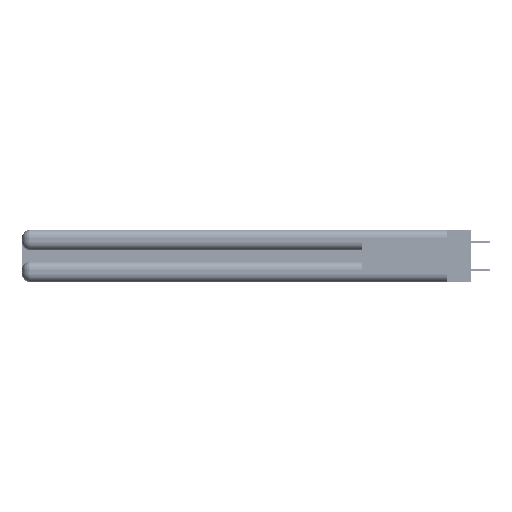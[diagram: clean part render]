
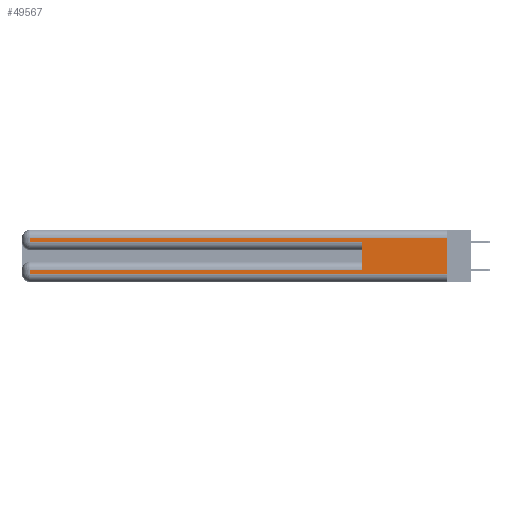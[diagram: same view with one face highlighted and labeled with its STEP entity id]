
A CAD part, left-side view. The second image highlights one B-rep face of the part: STEP entity #49567.
In plain terms, the highlighted planar face has unit normal (-1, 0, 0).
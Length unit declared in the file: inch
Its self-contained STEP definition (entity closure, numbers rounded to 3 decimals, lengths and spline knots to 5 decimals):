
#527 = VERTEX_POINT ( 'NONE', #23845 ) ;
#1686 = DIRECTION ( 'NONE',  ( 0., 1., 0. ) ) ;
#2031 = FACE_OUTER_BOUND ( 'NONE', #20656, .T. ) ;
#5132 = DIRECTION ( 'NONE',  ( 0., -1., 0. ) ) ;
#6232 = LINE ( 'NONE', #6499, #11793 ) ;
#6499 = CARTESIAN_POINT ( 'NONE',  ( 0., 0., 0.31 ) ) ;
#7122 = VERTEX_POINT ( 'NONE', #25408 ) ;
#7127 = CARTESIAN_POINT ( 'NONE',  ( 0., 0., 0.37 ) ) ;
#7706 = DIRECTION ( 'NONE',  ( 0., 1., 0. ) ) ;
#8809 = LINE ( 'NONE', #55264, #35926 ) ;
#9026 = ORIENTED_EDGE ( 'NONE', *, *, #32022, .F. ) ;
#10526 = CARTESIAN_POINT ( 'NONE',  ( 0., 0.6, 0.285 ) ) ;
#11391 = ORIENTED_EDGE ( 'NONE', *, *, #53715, .T. ) ;
#11528 = LINE ( 'NONE', #23981, #28652 ) ;
#11734 = VECTOR ( 'NONE', #44855, 39.37008 ) ;
#11793 = VECTOR ( 'NONE', #1686, 39.37008 ) ;
#11884 = CARTESIAN_POINT ( 'NONE',  ( 0., 0., 0.37 ) ) ;
#12085 = VERTEX_POINT ( 'NONE', #18252 ) ;
#12910 = LINE ( 'NONE', #13932, #48203 ) ;
#13932 = CARTESIAN_POINT ( 'NONE',  ( 0., 0., 0.285 ) ) ;
#14087 = CARTESIAN_POINT ( 'NONE',  ( 0., 2.94, 0.085 ) ) ;
#14174 = CARTESIAN_POINT ( 'NONE',  ( 0., 0., 0.06 ) ) ;
#14589 = CARTESIAN_POINT ( 'NONE',  ( 0., 0.6, 0.145 ) ) ;
#15603 = LINE ( 'NONE', #55485, #38259 ) ;
#17709 = EDGE_CURVE ( 'NONE', #24089, #52667, #27595, .T. ) ;
#18252 = CARTESIAN_POINT ( 'NONE',  ( 0., 2.94, 0.06 ) ) ;
#20656 = EDGE_LOOP ( 'NONE', ( #9026, #34301, #11391, #23757, #26245, #27391, #32848, #41834 ) ) ;
#21561 = VERTEX_POINT ( 'NONE', #14087 ) ;
#22673 = CARTESIAN_POINT ( 'NONE',  ( 0., 0.6, 0.085 ) ) ;
#23757 = ORIENTED_EDGE ( 'NONE', *, *, #49442, .T. ) ;
#23845 = CARTESIAN_POINT ( 'NONE',  ( 0., 2.94, 0.285 ) ) ;
#23981 = CARTESIAN_POINT ( 'NONE',  ( 0., 2.94, 0.37 ) ) ;
#24077 = EDGE_CURVE ( 'NONE', #12085, #7122, #26361, .T. ) ;
#24089 = VERTEX_POINT ( 'NONE', #22673 ) ;
#25141 = CARTESIAN_POINT ( 'NONE',  ( 0., 0., 0.31 ) ) ;
#25408 = CARTESIAN_POINT ( 'NONE',  ( 0., 0., 0.06 ) ) ;
#26245 = ORIENTED_EDGE ( 'NONE', *, *, #17709, .F. ) ;
#26361 = LINE ( 'NONE', #14174, #27383 ) ;
#27383 = VECTOR ( 'NONE', #5132, 39.37008 ) ;
#27391 = ORIENTED_EDGE ( 'NONE', *, *, #33366, .T. ) ;
#27595 = LINE ( 'NONE', #14589, #11734 ) ;
#28627 = PLANE ( 'NONE',  #33779 ) ;
#28652 = VECTOR ( 'NONE', #50009, 39.37008 ) ;
#29133 = DIRECTION ( 'NONE',  ( 0., 0., -1. ) ) ;
#31171 = DIRECTION ( 'NONE',  ( 0., -1., 0. ) ) ;
#32022 = EDGE_CURVE ( 'NONE', #35459, #7122, #50654, .T. ) ;
#32848 = ORIENTED_EDGE ( 'NONE', *, *, #47241, .T. ) ;
#33366 = EDGE_CURVE ( 'NONE', #24089, #21561, #8809, .T. ) ;
#33779 = AXIS2_PLACEMENT_3D ( 'NONE', #7127, #53837, #41633 ) ;
#34301 = ORIENTED_EDGE ( 'NONE', *, *, #37969, .T. ) ;
#35459 = VERTEX_POINT ( 'NONE', #25141 ) ;
#35926 = VECTOR ( 'NONE', #7706, 39.37008 ) ;
#37969 = EDGE_CURVE ( 'NONE', #35459, #51095, #6232, .T. ) ;
#38259 = VECTOR ( 'NONE', #51238, 39.37008 ) ;
#41633 = DIRECTION ( 'NONE',  ( 0., 0., -1. ) ) ;
#41834 = ORIENTED_EDGE ( 'NONE', *, *, #24077, .T. ) ;
#44855 = DIRECTION ( 'NONE',  ( 0., 0., 1. ) ) ;
#47241 = EDGE_CURVE ( 'NONE', #21561, #12085, #15603, .T. ) ;
#48203 = VECTOR ( 'NONE', #31171, 39.37008 ) ;
#49442 = EDGE_CURVE ( 'NONE', #527, #52667, #12910, .T. ) ;
#49567 = ADVANCED_FACE ( 'NONE', ( #2031 ), #28627, .F. ) ;
#50009 = DIRECTION ( 'NONE',  ( 0., 0., -1. ) ) ;
#50654 = LINE ( 'NONE', #11884, #53983 ) ;
#51095 = VERTEX_POINT ( 'NONE', #55010 ) ;
#51238 = DIRECTION ( 'NONE',  ( 0., 0., -1. ) ) ;
#52667 = VERTEX_POINT ( 'NONE', #10526 ) ;
#53715 = EDGE_CURVE ( 'NONE', #51095, #527, #11528, .T. ) ;
#53837 = DIRECTION ( 'NONE',  ( 1., 0., 0. ) ) ;
#53983 = VECTOR ( 'NONE', #29133, 39.37008 ) ;
#55010 = CARTESIAN_POINT ( 'NONE',  ( 0., 2.94, 0.31 ) ) ;
#55264 = CARTESIAN_POINT ( 'NONE',  ( 0., 0., 0.085 ) ) ;
#55485 = CARTESIAN_POINT ( 'NONE',  ( 0., 2.94, 0.37 ) ) ;
